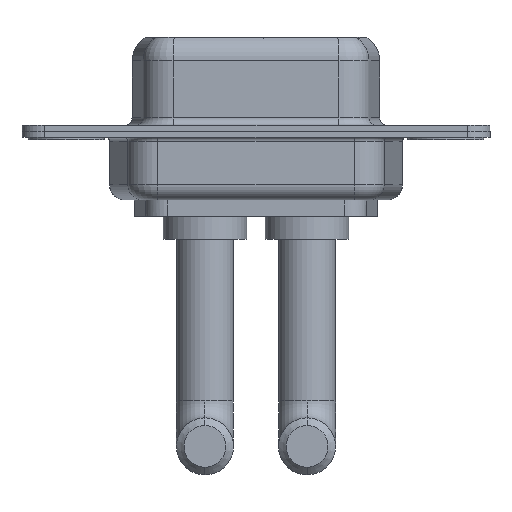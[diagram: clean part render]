
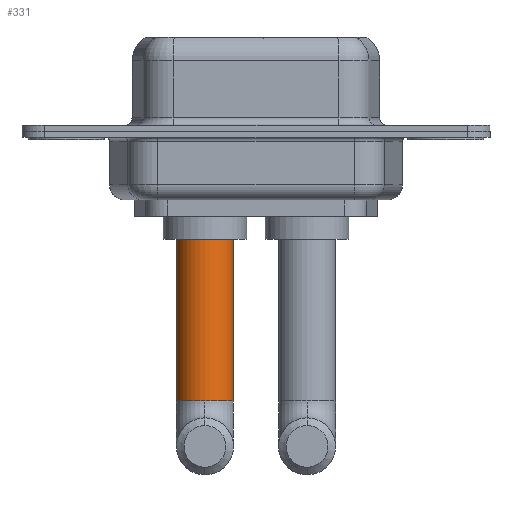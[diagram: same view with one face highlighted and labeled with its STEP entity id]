
A CAD part, front view. The second image highlights one B-rep face of the part: STEP entity #331.
In plain terms, the highlighted cylindrical face has radius 1.875 mm (diameter 3.75 mm), a partial arc.
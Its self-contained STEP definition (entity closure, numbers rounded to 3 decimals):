
#331 = ADVANCED_FACE ( 'NONE', ( #9930 ), #1944, .T. ) ;
#409 = CARTESIAN_POINT ( 'NONE',  ( 1.875, 0., -10.63 ) ) ;
#681 = CARTESIAN_POINT ( 'NONE',  ( -1.875, 0., 0. ) ) ;
#1012 = DIRECTION ( 'NONE',  ( 0., 0., -1. ) ) ;
#1014 = AXIS2_PLACEMENT_3D ( 'NONE', #4817, #3000, #2119 ) ;
#1441 = CARTESIAN_POINT ( 'NONE',  ( 1.875, 0., 0. ) ) ;
#1484 = VECTOR ( 'NONE', #11241, 1000. ) ;
#1631 = ORIENTED_EDGE ( 'NONE', *, *, #6065, .F. ) ;
#1758 = AXIS2_PLACEMENT_3D ( 'NONE', #4176, #5997, #7728 ) ;
#1944 = CYLINDRICAL_SURFACE ( 'NONE', #7309, 1.875 ) ;
#2119 = DIRECTION ( 'NONE',  ( -1., 0., 0. ) ) ;
#2938 = CARTESIAN_POINT ( 'NONE',  ( 0., 0., 0. ) ) ;
#3000 = DIRECTION ( 'NONE',  ( 0., 0., -1. ) ) ;
#3117 = VERTEX_POINT ( 'NONE', #6466 ) ;
#3184 = CARTESIAN_POINT ( 'NONE',  ( -1.875, 0., 0. ) ) ;
#3201 = VERTEX_POINT ( 'NONE', #1441 ) ;
#3625 = DIRECTION ( 'NONE',  ( -1., 0., 0. ) ) ;
#3888 = VERTEX_POINT ( 'NONE', #409 ) ;
#4176 = CARTESIAN_POINT ( 'NONE',  ( 0., 0., 0. ) ) ;
#4817 = CARTESIAN_POINT ( 'NONE',  ( 0., 0., -10.63 ) ) ;
#5559 = LINE ( 'NONE', #10984, #11006 ) ;
#5997 = DIRECTION ( 'NONE',  ( 0., 0., -1. ) ) ;
#6065 = EDGE_CURVE ( 'NONE', #3117, #9888, #10353, .T. ) ;
#6466 = CARTESIAN_POINT ( 'NONE',  ( 0., -1.875, -10.63 ) ) ;
#6502 = DIRECTION ( 'NONE',  ( -1., 0., 0. ) ) ;
#6686 = EDGE_CURVE ( 'NONE', #3201, #8491, #6796, .T. ) ;
#6796 = CIRCLE ( 'NONE', #1758, 1.875 ) ;
#6854 = EDGE_CURVE ( 'NONE', #3888, #3117, #10343, .T. ) ;
#7309 = AXIS2_PLACEMENT_3D ( 'NONE', #2938, #1012, #6502 ) ;
#7728 = DIRECTION ( 'NONE',  ( -1., 0., 0. ) ) ;
#8231 = DIRECTION ( 'NONE',  ( 0., 0., -1. ) ) ;
#8491 = VERTEX_POINT ( 'NONE', #3184 ) ;
#8500 = ORIENTED_EDGE ( 'NONE', *, *, #6686, .T. ) ;
#8541 = CARTESIAN_POINT ( 'NONE',  ( -1.875, 0., -10.63 ) ) ;
#8656 = ORIENTED_EDGE ( 'NONE', *, *, #6854, .F. ) ;
#9105 = DIRECTION ( 'NONE',  ( 0., 0., -1. ) ) ;
#9422 = EDGE_CURVE ( 'NONE', #8491, #9888, #10196, .T. ) ;
#9605 = AXIS2_PLACEMENT_3D ( 'NONE', #9810, #8231, #3625 ) ;
#9735 = ORIENTED_EDGE ( 'NONE', *, *, #11357, .F. ) ;
#9810 = CARTESIAN_POINT ( 'NONE',  ( 0., 0., -10.63 ) ) ;
#9888 = VERTEX_POINT ( 'NONE', #8541 ) ;
#9930 = FACE_OUTER_BOUND ( 'NONE', #10769, .T. ) ;
#10196 = LINE ( 'NONE', #681, #1484 ) ;
#10343 = CIRCLE ( 'NONE', #1014, 1.875 ) ;
#10353 = CIRCLE ( 'NONE', #9605, 1.875 ) ;
#10769 = EDGE_LOOP ( 'NONE', ( #9735, #8500, #10914, #1631, #8656 ) ) ;
#10914 = ORIENTED_EDGE ( 'NONE', *, *, #9422, .T. ) ;
#10984 = CARTESIAN_POINT ( 'NONE',  ( 1.875, 0., 0. ) ) ;
#11006 = VECTOR ( 'NONE', #9105, 1000. ) ;
#11241 = DIRECTION ( 'NONE',  ( 0., 0., -1. ) ) ;
#11357 = EDGE_CURVE ( 'NONE', #3201, #3888, #5559, .T. ) ;
